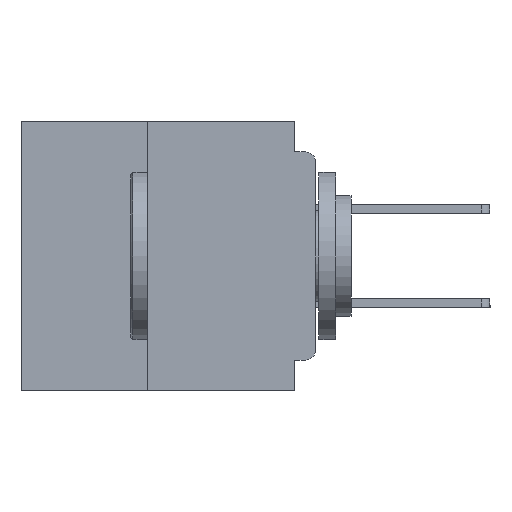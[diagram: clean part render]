
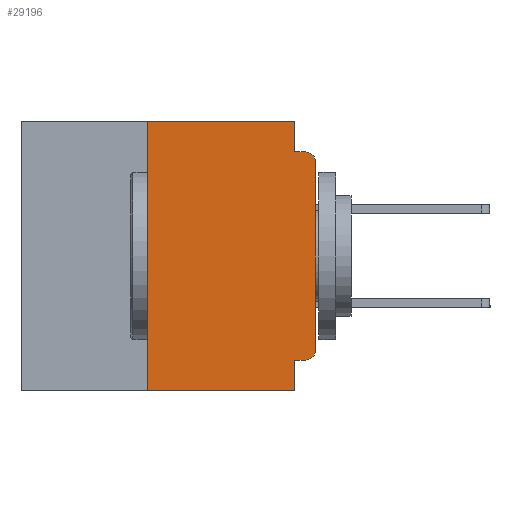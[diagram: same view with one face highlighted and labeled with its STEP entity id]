
A CAD part, left-side view. The second image highlights one B-rep face of the part: STEP entity #29196.
In plain terms, the highlighted planar face has unit normal (-1, 0, 0).
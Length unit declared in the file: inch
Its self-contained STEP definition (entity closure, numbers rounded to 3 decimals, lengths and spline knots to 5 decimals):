
#214 = LINE ( 'NONE', #28739, #16064 ) ;
#1090 = VECTOR ( 'NONE', #30600, 39.37008 ) ;
#1545 = DIRECTION ( 'NONE',  ( -1., 0., 0. ) ) ;
#1927 = ORIENTED_EDGE ( 'NONE', *, *, #25727, .F. ) ;
#2194 = LINE ( 'NONE', #33416, #24815 ) ;
#2244 = VERTEX_POINT ( 'NONE', #28212 ) ;
#2452 = CARTESIAN_POINT ( 'NONE',  ( 0., 0.015, -0.355 ) ) ;
#2970 = ORIENTED_EDGE ( 'NONE', *, *, #35356, .F. ) ;
#3051 = ORIENTED_EDGE ( 'NONE', *, *, #29188, .T. ) ;
#3466 = CARTESIAN_POINT ( 'NONE',  ( 0., 0., 0. ) ) ;
#4156 = DIRECTION ( 'NONE',  ( 0., 0., -1. ) ) ;
#4781 = PLANE ( 'NONE',  #34804 ) ;
#4800 = CARTESIAN_POINT ( 'NONE',  ( 0., 0.437, -0.4 ) ) ;
#4952 = CARTESIAN_POINT ( 'NONE',  ( 0., 0.25, 0. ) ) ;
#5041 = AXIS2_PLACEMENT_3D ( 'NONE', #19332, #1545, #22239 ) ;
#5432 = CARTESIAN_POINT ( 'NONE',  ( 0., 0.25, -0.4 ) ) ;
#5454 = ORIENTED_EDGE ( 'NONE', *, *, #18742, .F. ) ;
#5688 = FACE_OUTER_BOUND ( 'NONE', #24420, .T. ) ;
#5699 = CARTESIAN_POINT ( 'NONE',  ( 0., 0.015, -0.045 ) ) ;
#5705 = VECTOR ( 'NONE', #16581, 39.37008 ) ;
#6435 = ORIENTED_EDGE ( 'NONE', *, *, #33021, .T. ) ;
#6528 = VECTOR ( 'NONE', #33975, 39.37008 ) ;
#6646 = LINE ( 'NONE', #4800, #5705 ) ;
#6869 = EDGE_CURVE ( 'NONE', #8142, #18373, #17870, .T. ) ;
#7902 = EDGE_CURVE ( 'NONE', #28724, #18466, #28737, .T. ) ;
#8142 = VERTEX_POINT ( 'NONE', #2452 ) ;
#9153 = CARTESIAN_POINT ( 'NONE',  ( 0., 0.031, 0. ) ) ;
#10651 = DIRECTION ( 'NONE',  ( 0., -1., 0. ) ) ;
#10716 = CARTESIAN_POINT ( 'NONE',  ( 0., 0.437, 0. ) ) ;
#10925 = CARTESIAN_POINT ( 'NONE',  ( 0., 0.437, 0. ) ) ;
#11216 = DIRECTION ( 'NONE',  ( 0., 0., -1. ) ) ;
#13714 = DIRECTION ( 'NONE',  ( -1., 0., 0. ) ) ;
#14086 = CARTESIAN_POINT ( 'NONE',  ( 0., 0.25, -0.4 ) ) ;
#14612 = ORIENTED_EDGE ( 'NONE', *, *, #23782, .T. ) ;
#15675 = VERTEX_POINT ( 'NONE', #19715 ) ;
#16064 = VECTOR ( 'NONE', #11216, 39.37008 ) ;
#16243 = LINE ( 'NONE', #31107, #6528 ) ;
#16581 = DIRECTION ( 'NONE',  ( 0., -1., 0. ) ) ;
#16689 = DIRECTION ( 'NONE',  ( 1., 0., 0. ) ) ;
#17806 = VERTEX_POINT ( 'NONE', #5699 ) ;
#17870 = LINE ( 'NONE', #27157, #1090 ) ;
#18373 = VERTEX_POINT ( 'NONE', #29128 ) ;
#18466 = VERTEX_POINT ( 'NONE', #9153 ) ;
#18742 = EDGE_CURVE ( 'NONE', #15675, #17806, #16243, .T. ) ;
#19332 = CARTESIAN_POINT ( 'NONE',  ( 0., 0.015, -0.06 ) ) ;
#19715 = CARTESIAN_POINT ( 'NONE',  ( 0., 0.031, -0.045 ) ) ;
#20529 = ORIENTED_EDGE ( 'NONE', *, *, #6869, .F. ) ;
#21842 = EDGE_CURVE ( 'NONE', #18373, #32045, #214, .T. ) ;
#21860 = CARTESIAN_POINT ( 'NONE',  ( 0., 0., -0.34 ) ) ;
#22237 = VERTEX_POINT ( 'NONE', #21860 ) ;
#22239 = DIRECTION ( 'NONE',  ( 0., 0., -1. ) ) ;
#22405 = ORIENTED_EDGE ( 'NONE', *, *, #7902, .F. ) ;
#23782 = EDGE_CURVE ( 'NONE', #33875, #32045, #6646, .T. ) ;
#24420 = EDGE_LOOP ( 'NONE', ( #29569, #6435, #5454, #2970, #22405, #1927, #14612, #31244, #20529, #3051 ) ) ;
#24815 = VECTOR ( 'NONE', #4156, 39.37008 ) ;
#25352 = VECTOR ( 'NONE', #37247, 39.37008 ) ;
#25727 = EDGE_CURVE ( 'NONE', #33875, #28724, #33029, .T. ) ;
#26998 = DIRECTION ( 'NONE',  ( 0., 0., 1. ) ) ;
#27097 = AXIS2_PLACEMENT_3D ( 'NONE', #31150, #13714, #34029 ) ;
#27157 = CARTESIAN_POINT ( 'NONE',  ( 0., 0., -0.355 ) ) ;
#27831 = VECTOR ( 'NONE', #10651, 39.37008 ) ;
#28212 = CARTESIAN_POINT ( 'NONE',  ( 0., 0., -0.06 ) ) ;
#28724 = VERTEX_POINT ( 'NONE', #4952 ) ;
#28737 = LINE ( 'NONE', #10925, #27831 ) ;
#28739 = CARTESIAN_POINT ( 'NONE',  ( 0., 0.031, -0.4 ) ) ;
#29084 = CIRCLE ( 'NONE', #27097, 0.015 ) ;
#29128 = CARTESIAN_POINT ( 'NONE',  ( 0., 0.031, -0.355 ) ) ;
#29188 = EDGE_CURVE ( 'NONE', #8142, #22237, #29084, .T. ) ;
#29196 = ADVANCED_FACE ( 'NONE', ( #5688 ), #4781, .F. ) ;
#29569 = ORIENTED_EDGE ( 'NONE', *, *, #32306, .T. ) ;
#30420 = CIRCLE ( 'NONE', #5041, 0.015 ) ;
#30600 = DIRECTION ( 'NONE',  ( 0., 1., 0. ) ) ;
#31107 = CARTESIAN_POINT ( 'NONE',  ( 0., 0., -0.045 ) ) ;
#31150 = CARTESIAN_POINT ( 'NONE',  ( 0., 0.015, -0.34 ) ) ;
#31244 = ORIENTED_EDGE ( 'NONE', *, *, #21842, .F. ) ;
#31414 = CARTESIAN_POINT ( 'NONE',  ( 0., 0.031, -0.4 ) ) ;
#32045 = VERTEX_POINT ( 'NONE', #31414 ) ;
#32306 = EDGE_CURVE ( 'NONE', #22237, #2244, #35415, .T. ) ;
#33021 = EDGE_CURVE ( 'NONE', #2244, #17806, #30420, .T. ) ;
#33029 = LINE ( 'NONE', #14086, #25352 ) ;
#33416 = CARTESIAN_POINT ( 'NONE',  ( 0., 0.031, 0. ) ) ;
#33643 = VECTOR ( 'NONE', #26998, 39.37008 ) ;
#33875 = VERTEX_POINT ( 'NONE', #5432 ) ;
#33975 = DIRECTION ( 'NONE',  ( 0., -1., 0. ) ) ;
#34029 = DIRECTION ( 'NONE',  ( 0., 0., -1. ) ) ;
#34804 = AXIS2_PLACEMENT_3D ( 'NONE', #10716, #16689, #36888 ) ;
#35356 = EDGE_CURVE ( 'NONE', #18466, #15675, #2194, .T. ) ;
#35415 = LINE ( 'NONE', #3466, #33643 ) ;
#36888 = DIRECTION ( 'NONE',  ( 0., 0., -1. ) ) ;
#37247 = DIRECTION ( 'NONE',  ( 0., 0., 1. ) ) ;
